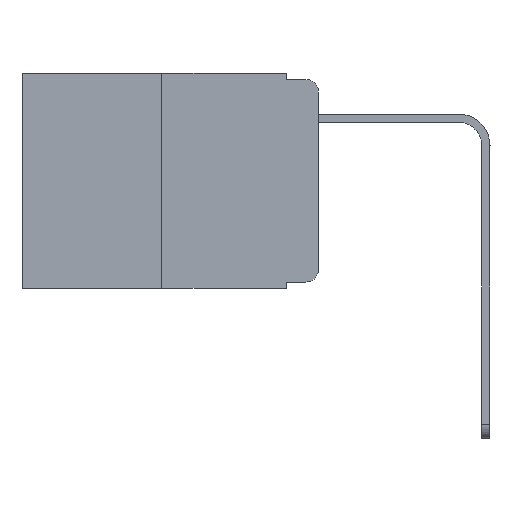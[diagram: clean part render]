
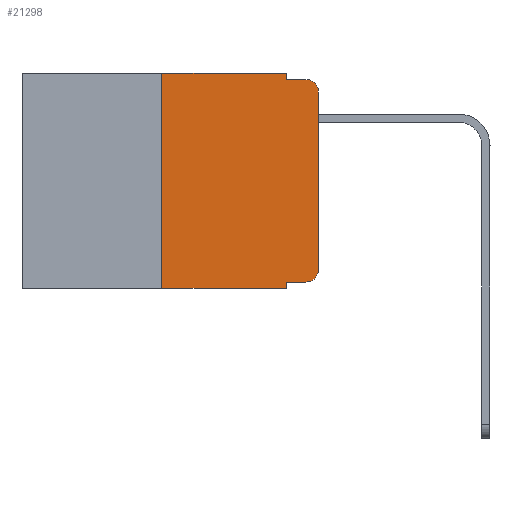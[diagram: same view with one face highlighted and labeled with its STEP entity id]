
A CAD part, left-side view. The second image highlights one B-rep face of the part: STEP entity #21298.
In plain terms, the highlighted planar face has unit normal (-1, 0, 0).
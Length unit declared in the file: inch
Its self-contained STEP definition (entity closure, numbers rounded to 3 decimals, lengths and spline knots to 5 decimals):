
#31 = DIRECTION ( 'NONE',  ( 1., 0., 0. ) ) ;
#52 = VECTOR ( 'NONE', #17337, 39.37008 ) ;
#85 = ORIENTED_EDGE ( 'NONE', *, *, #17824, .F. ) ;
#97 = DIRECTION ( 'NONE',  ( -1., 0., 0. ) ) ;
#272 = EDGE_CURVE ( 'NONE', #21878, #20878, #17976, .T. ) ;
#494 = LINE ( 'NONE', #15008, #6403 ) ;
#735 = EDGE_CURVE ( 'NONE', #4387, #18090, #2982, .T. ) ;
#1317 = VERTEX_POINT ( 'NONE', #11679 ) ;
#1329 = AXIS2_PLACEMENT_3D ( 'NONE', #10310, #10386, #10467 ) ;
#1631 = CARTESIAN_POINT ( 'NONE',  ( 0., 0.051, 0. ) ) ;
#1770 = CARTESIAN_POINT ( 'NONE',  ( 0., 0.02, -0.01 ) ) ;
#2020 = EDGE_CURVE ( 'NONE', #1317, #21436, #20832, .T. ) ;
#2547 = CIRCLE ( 'NONE', #13597, 0.02 ) ;
#2982 = CIRCLE ( 'NONE', #1329, 0.02 ) ;
#3066 = CARTESIAN_POINT ( 'NONE',  ( 0., 0., -0.03 ) ) ;
#3397 = CARTESIAN_POINT ( 'NONE',  ( 0., 0.473, 0. ) ) ;
#3531 = VECTOR ( 'NONE', #14716, 39.37008 ) ;
#3544 = EDGE_CURVE ( 'NONE', #16789, #13138, #2547, .T. ) ;
#3650 = ORIENTED_EDGE ( 'NONE', *, *, #9246, .F. ) ;
#3724 = CARTESIAN_POINT ( 'NONE',  ( 0., 0., 0. ) ) ;
#3920 = VERTEX_POINT ( 'NONE', #5584 ) ;
#3930 = ORIENTED_EDGE ( 'NONE', *, *, #272, .F. ) ;
#4387 = VERTEX_POINT ( 'NONE', #21808 ) ;
#4574 = LINE ( 'NONE', #19204, #52 ) ;
#4814 = ORIENTED_EDGE ( 'NONE', *, *, #5767, .F. ) ;
#5584 = CARTESIAN_POINT ( 'NONE',  ( 0., 0.25, 0. ) ) ;
#5605 = EDGE_LOOP ( 'NONE', ( #21403, #18248, #4814, #3930, #3650, #85, #12182, #18213, #11070, #6531 ) ) ;
#5767 = EDGE_CURVE ( 'NONE', #20878, #13138, #19414, .T. ) ;
#6403 = VECTOR ( 'NONE', #13622, 39.37008 ) ;
#6531 = ORIENTED_EDGE ( 'NONE', *, *, #735, .T. ) ;
#6605 = CARTESIAN_POINT ( 'NONE',  ( 0., 0., -0.313 ) ) ;
#6620 = LINE ( 'NONE', #3724, #19159 ) ;
#6772 = VECTOR ( 'NONE', #22126, 39.37008 ) ;
#7839 = LINE ( 'NONE', #16071, #10536 ) ;
#8701 = DIRECTION ( 'NONE',  ( 0., 0., -1. ) ) ;
#9246 = EDGE_CURVE ( 'NONE', #3920, #21878, #21985, .T. ) ;
#9326 = CARTESIAN_POINT ( 'NONE',  ( 0., 0.051, -0.01 ) ) ;
#10189 = CARTESIAN_POINT ( 'NONE',  ( 0., 0.051, 0. ) ) ;
#10310 = CARTESIAN_POINT ( 'NONE',  ( 0., 0.02, -0.313 ) ) ;
#10386 = DIRECTION ( 'NONE',  ( -1., 0., 0. ) ) ;
#10467 = DIRECTION ( 'NONE',  ( 0., 0., -1. ) ) ;
#10536 = VECTOR ( 'NONE', #12608, 39.37008 ) ;
#11070 = ORIENTED_EDGE ( 'NONE', *, *, #20566, .T. ) ;
#11186 = FACE_OUTER_BOUND ( 'NONE', #5605, .T. ) ;
#11368 = EDGE_CURVE ( 'NONE', #18090, #16789, #6620, .T. ) ;
#11664 = CARTESIAN_POINT ( 'NONE',  ( 0., 0.473, -0.343 ) ) ;
#11679 = CARTESIAN_POINT ( 'NONE',  ( 0., 0.25, -0.343 ) ) ;
#12182 = ORIENTED_EDGE ( 'NONE', *, *, #2020, .T. ) ;
#12365 = DIRECTION ( 'NONE',  ( 0., 0., 1. ) ) ;
#12608 = DIRECTION ( 'NONE',  ( 0., 0., 1. ) ) ;
#13105 = CARTESIAN_POINT ( 'NONE',  ( 0., 0.473, 0. ) ) ;
#13138 = VERTEX_POINT ( 'NONE', #1770 ) ;
#13523 = PLANE ( 'NONE',  #18198 ) ;
#13597 = AXIS2_PLACEMENT_3D ( 'NONE', #18836, #97, #8701 ) ;
#13622 = DIRECTION ( 'NONE',  ( 0., -1., 0. ) ) ;
#13672 = DIRECTION ( 'NONE',  ( 0., 0., -1. ) ) ;
#14716 = DIRECTION ( 'NONE',  ( 0., -1., 0. ) ) ;
#15008 = CARTESIAN_POINT ( 'NONE',  ( 0., 0.051, -0.333 ) ) ;
#15681 = VECTOR ( 'NONE', #18661, 39.37008 ) ;
#15856 = CARTESIAN_POINT ( 'NONE',  ( 0., 0.051, -0.333 ) ) ;
#16071 = CARTESIAN_POINT ( 'NONE',  ( 0., 0.25, 0. ) ) ;
#16789 = VERTEX_POINT ( 'NONE', #3066 ) ;
#17337 = DIRECTION ( 'NONE',  ( 0., 0., -1. ) ) ;
#17355 = CARTESIAN_POINT ( 'NONE',  ( 0., 0.051, -0.343 ) ) ;
#17824 = EDGE_CURVE ( 'NONE', #1317, #3920, #7839, .T. ) ;
#17976 = LINE ( 'NONE', #10189, #6772 ) ;
#18090 = VERTEX_POINT ( 'NONE', #6605 ) ;
#18198 = AXIS2_PLACEMENT_3D ( 'NONE', #3397, #31, #13672 ) ;
#18213 = ORIENTED_EDGE ( 'NONE', *, *, #18293, .F. ) ;
#18248 = ORIENTED_EDGE ( 'NONE', *, *, #3544, .T. ) ;
#18293 = EDGE_CURVE ( 'NONE', #21519, #21436, #4574, .T. ) ;
#18661 = DIRECTION ( 'NONE',  ( 0., -1., 0. ) ) ;
#18698 = VECTOR ( 'NONE', #21644, 39.37008 ) ;
#18836 = CARTESIAN_POINT ( 'NONE',  ( 0., 0.02, -0.03 ) ) ;
#19159 = VECTOR ( 'NONE', #12365, 39.37008 ) ;
#19204 = CARTESIAN_POINT ( 'NONE',  ( 0., 0.051, 0. ) ) ;
#19414 = LINE ( 'NONE', #21500, #15681 ) ;
#20566 = EDGE_CURVE ( 'NONE', #21519, #4387, #494, .T. ) ;
#20832 = LINE ( 'NONE', #11664, #18698 ) ;
#20878 = VERTEX_POINT ( 'NONE', #9326 ) ;
#21298 = ADVANCED_FACE ( 'NONE', ( #11186 ), #13523, .F. ) ;
#21403 = ORIENTED_EDGE ( 'NONE', *, *, #11368, .T. ) ;
#21436 = VERTEX_POINT ( 'NONE', #17355 ) ;
#21500 = CARTESIAN_POINT ( 'NONE',  ( 0., 0.051, -0.01 ) ) ;
#21519 = VERTEX_POINT ( 'NONE', #15856 ) ;
#21644 = DIRECTION ( 'NONE',  ( 0., -1., 0. ) ) ;
#21808 = CARTESIAN_POINT ( 'NONE',  ( 0., 0.02, -0.333 ) ) ;
#21878 = VERTEX_POINT ( 'NONE', #1631 ) ;
#21985 = LINE ( 'NONE', #13105, #3531 ) ;
#22126 = DIRECTION ( 'NONE',  ( 0., 0., -1. ) ) ;
